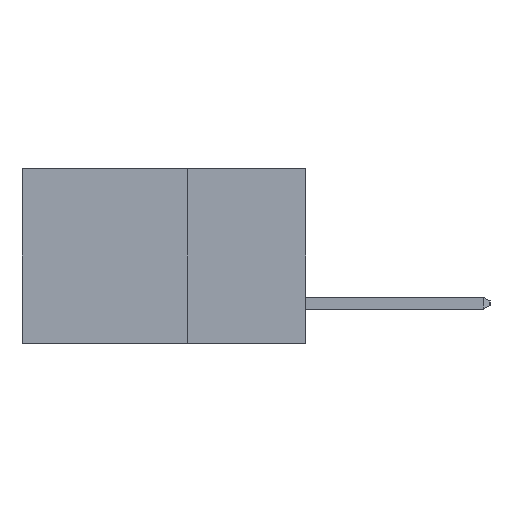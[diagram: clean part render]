
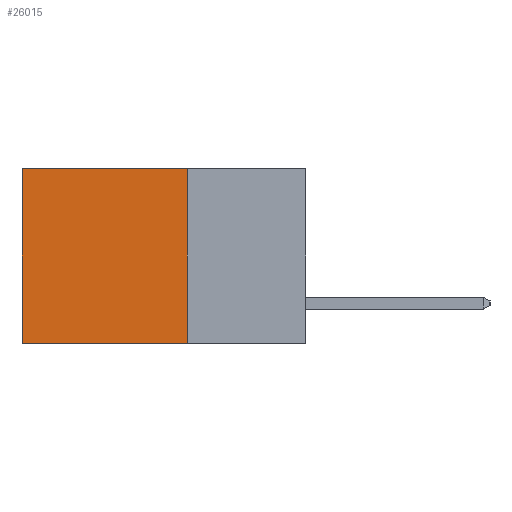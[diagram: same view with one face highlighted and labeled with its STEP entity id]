
A CAD part, left-side view. The second image highlights one B-rep face of the part: STEP entity #26015.
In plain terms, the highlighted planar face has unit normal (-1, 0, 0).
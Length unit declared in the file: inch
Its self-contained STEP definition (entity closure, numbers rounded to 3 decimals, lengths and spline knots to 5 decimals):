
#305 = CARTESIAN_POINT ( 'NONE',  ( 0.298, 0.6, 0. ) ) ;
#381 = VERTEX_POINT ( 'NONE', #22122 ) ;
#2864 = ORIENTED_EDGE ( 'NONE', *, *, #28499, .F. ) ;
#3503 = LINE ( 'NONE', #24196, #20579 ) ;
#3806 = VECTOR ( 'NONE', #14088, 39.37008 ) ;
#4661 = DIRECTION ( 'NONE',  ( 0., 0., -1. ) ) ;
#6045 = ORIENTED_EDGE ( 'NONE', *, *, #28172, .F. ) ;
#6639 = VECTOR ( 'NONE', #23163, 39.37008 ) ;
#7994 = DIRECTION ( 'NONE',  ( 0., 0., -1. ) ) ;
#8958 = LINE ( 'NONE', #27342, #3806 ) ;
#9436 = VERTEX_POINT ( 'NONE', #19183 ) ;
#10532 = CARTESIAN_POINT ( 'NONE',  ( 0.298, 0.25, 0. ) ) ;
#11459 = LINE ( 'NONE', #17988, #18824 ) ;
#12328 = EDGE_LOOP ( 'NONE', ( #13537, #6045, #2864, #18234 ) ) ;
#12539 = LINE ( 'NONE', #27411, #6639 ) ;
#13537 = ORIENTED_EDGE ( 'NONE', *, *, #21593, .T. ) ;
#13977 = FACE_OUTER_BOUND ( 'NONE', #12328, .T. ) ;
#14088 = DIRECTION ( 'NONE',  ( 0., 0., -1. ) ) ;
#14270 = VERTEX_POINT ( 'NONE', #10532 ) ;
#16889 = PLANE ( 'NONE',  #27524 ) ;
#17867 = VERTEX_POINT ( 'NONE', #305 ) ;
#17988 = CARTESIAN_POINT ( 'NONE',  ( 0.298, 0.25, 0. ) ) ;
#18234 = ORIENTED_EDGE ( 'NONE', *, *, #27836, .T. ) ;
#18824 = VECTOR ( 'NONE', #4661, 39.37008 ) ;
#19157 = CARTESIAN_POINT ( 'NONE',  ( 0.298, 0.25, 0. ) ) ;
#19183 = CARTESIAN_POINT ( 'NONE',  ( 0.298, 0.6, -0.37 ) ) ;
#20579 = VECTOR ( 'NONE', #28447, 39.37008 ) ;
#21415 = DIRECTION ( 'NONE',  ( 1., 0., 0. ) ) ;
#21593 = EDGE_CURVE ( 'NONE', #17867, #9436, #8958, .T. ) ;
#22122 = CARTESIAN_POINT ( 'NONE',  ( 0.298, 0.25, -0.37 ) ) ;
#23163 = DIRECTION ( 'NONE',  ( 0., 1., 0. ) ) ;
#24196 = CARTESIAN_POINT ( 'NONE',  ( 0.298, 0.25, -0.37 ) ) ;
#26015 = ADVANCED_FACE ( 'NONE', ( #13977 ), #16889, .F. ) ;
#27342 = CARTESIAN_POINT ( 'NONE',  ( 0.298, 0.6, 0. ) ) ;
#27411 = CARTESIAN_POINT ( 'NONE',  ( 0.298, 0.25, 0. ) ) ;
#27524 = AXIS2_PLACEMENT_3D ( 'NONE', #19157, #21415, #7994 ) ;
#27836 = EDGE_CURVE ( 'NONE', #14270, #17867, #12539, .T. ) ;
#28172 = EDGE_CURVE ( 'NONE', #381, #9436, #3503, .T. ) ;
#28447 = DIRECTION ( 'NONE',  ( 0., 1., 0. ) ) ;
#28499 = EDGE_CURVE ( 'NONE', #14270, #381, #11459, .T. ) ;
